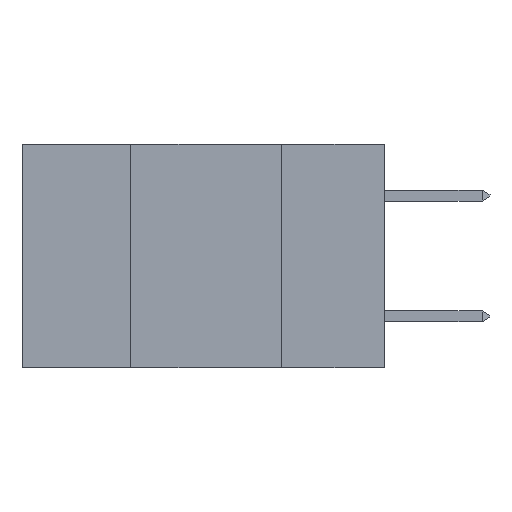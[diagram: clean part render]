
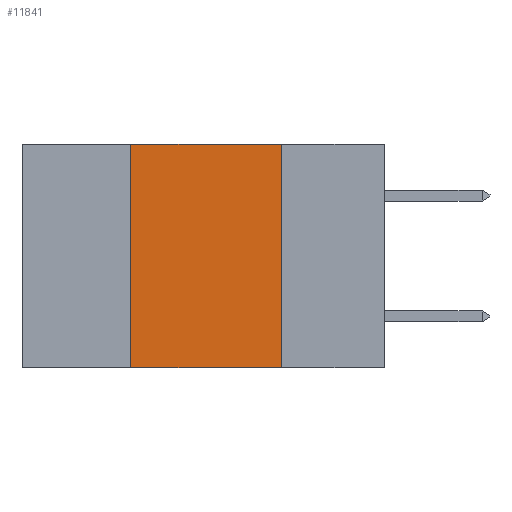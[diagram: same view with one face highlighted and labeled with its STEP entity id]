
A CAD part, left-side view. The second image highlights one B-rep face of the part: STEP entity #11841.
In plain terms, the highlighted planar face has unit normal (-1, 0, 0).
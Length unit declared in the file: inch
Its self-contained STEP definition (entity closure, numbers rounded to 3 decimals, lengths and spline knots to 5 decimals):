
#232 = DIRECTION ( 'NONE',  ( 0., -1., 0. ) ) ;
#715 = VERTEX_POINT ( 'NONE', #4918 ) ;
#940 = FACE_OUTER_BOUND ( 'NONE', #1301, .T. ) ;
#1301 = EDGE_LOOP ( 'NONE', ( #6760, #12192, #10945, #10809 ) ) ;
#1379 = CARTESIAN_POINT ( 'NONE',  ( 0., 0.17, -0.37 ) ) ;
#1502 = EDGE_CURVE ( 'NONE', #715, #10926, #8950, .T. ) ;
#1530 = DIRECTION ( 'NONE',  ( 1., 0., 0. ) ) ;
#2395 = DIRECTION ( 'NONE',  ( 0., 0., -1. ) ) ;
#2443 = VECTOR ( 'NONE', #232, 39.37008 ) ;
#3266 = CARTESIAN_POINT ( 'NONE',  ( 0., 0.6, -0.37 ) ) ;
#3380 = VERTEX_POINT ( 'NONE', #1379 ) ;
#3750 = LINE ( 'NONE', #7917, #9230 ) ;
#3917 = CARTESIAN_POINT ( 'NONE',  ( 0., 0.6, 0. ) ) ;
#4179 = PLANE ( 'NONE',  #8260 ) ;
#4918 = CARTESIAN_POINT ( 'NONE',  ( 0., 0.42, 0. ) ) ;
#5122 = DIRECTION ( 'NONE',  ( 0., 0., -1. ) ) ;
#5413 = CARTESIAN_POINT ( 'NONE',  ( 0., 0.42, -0.37 ) ) ;
#5420 = VECTOR ( 'NONE', #11913, 39.37008 ) ;
#5730 = LINE ( 'NONE', #10859, #5420 ) ;
#6077 = EDGE_CURVE ( 'NONE', #8888, #715, #5730, .T. ) ;
#6760 = ORIENTED_EDGE ( 'NONE', *, *, #9235, .F. ) ;
#7052 = CARTESIAN_POINT ( 'NONE',  ( 0., 0.6, 0. ) ) ;
#7546 = CARTESIAN_POINT ( 'NONE',  ( 0., 0.17, 0. ) ) ;
#7917 = CARTESIAN_POINT ( 'NONE',  ( 0., 0.17, 0. ) ) ;
#8260 = AXIS2_PLACEMENT_3D ( 'NONE', #7052, #1530, #2395 ) ;
#8888 = VERTEX_POINT ( 'NONE', #5413 ) ;
#8950 = LINE ( 'NONE', #3917, #9537 ) ;
#9230 = VECTOR ( 'NONE', #5122, 39.37008 ) ;
#9235 = EDGE_CURVE ( 'NONE', #10926, #3380, #3750, .T. ) ;
#9537 = VECTOR ( 'NONE', #11479, 39.37008 ) ;
#10809 = ORIENTED_EDGE ( 'NONE', *, *, #12046, .T. ) ;
#10859 = CARTESIAN_POINT ( 'NONE',  ( 0., 0.42, 0. ) ) ;
#10926 = VERTEX_POINT ( 'NONE', #7546 ) ;
#10945 = ORIENTED_EDGE ( 'NONE', *, *, #6077, .F. ) ;
#11467 = LINE ( 'NONE', #3266, #2443 ) ;
#11479 = DIRECTION ( 'NONE',  ( 0., -1., 0. ) ) ;
#11841 = ADVANCED_FACE ( 'NONE', ( #940 ), #4179, .F. ) ;
#11913 = DIRECTION ( 'NONE',  ( 0., 0., 1. ) ) ;
#12046 = EDGE_CURVE ( 'NONE', #8888, #3380, #11467, .T. ) ;
#12192 = ORIENTED_EDGE ( 'NONE', *, *, #1502, .F. ) ;
